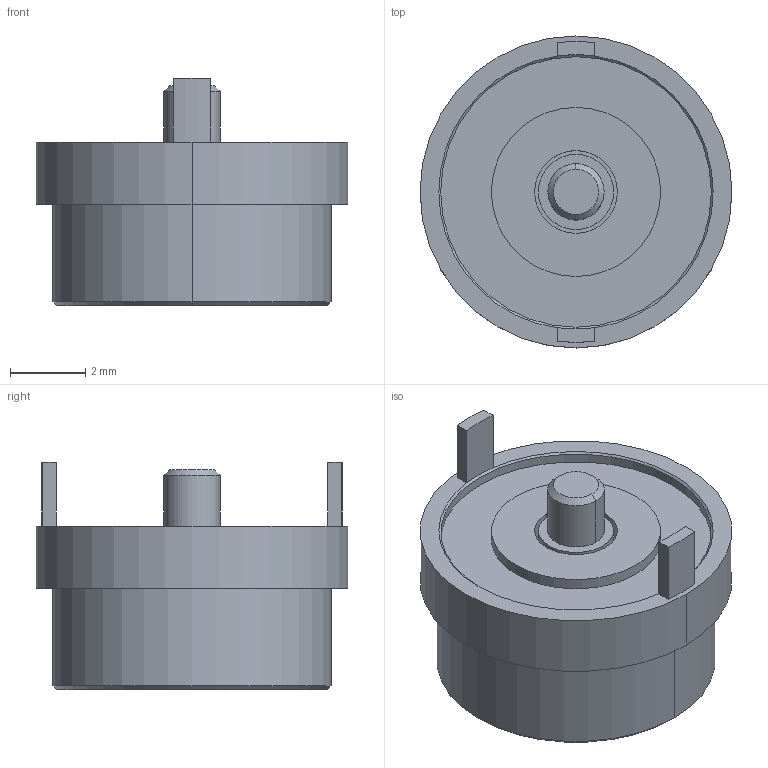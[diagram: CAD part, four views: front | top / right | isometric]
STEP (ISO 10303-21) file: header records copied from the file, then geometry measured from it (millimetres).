
FILE_DESCRIPTION (( 'STEP AP203' ), '1' );
FILE_NAME ('685-C02212021C1.STEP', '2023-02-02T10:17:16', ( '' ), ( '' ), 'SwSTEP 2.0', 'SolidWorks 2020', '' );
FILE_SCHEMA (( 'CONFIG_CONTROL_DESIGN' ));
Length unit declared in the file: millimetre
Products named in the file (1): 685-C02212021C1
Bounding box: 8.3 x 8.3 x 6.05 mm (x, y, z)
Volume: 195.3 mm3; surface area: 260.7 mm2
Topology: 1 solids, 1 shells, 53 faces, 114 edges, 71 vertices
Faces by surface type: cylinder 26, plane 16, cone 8, torus 2, sphere 1
Entity records: 1517 total; most frequent: DIRECTION 286, CARTESIAN_POINT 236, ORIENTED_EDGE 224, AXIS2_PLACEMENT_3D 120, EDGE_CURVE 112, VERTEX_POINT 70, CIRCLE 66, EDGE_LOOP 62
